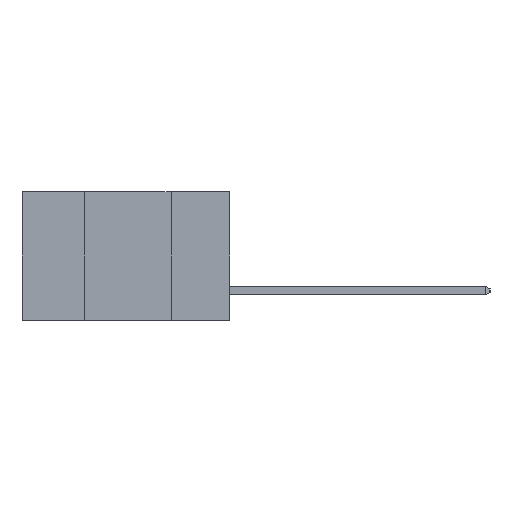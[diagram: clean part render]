
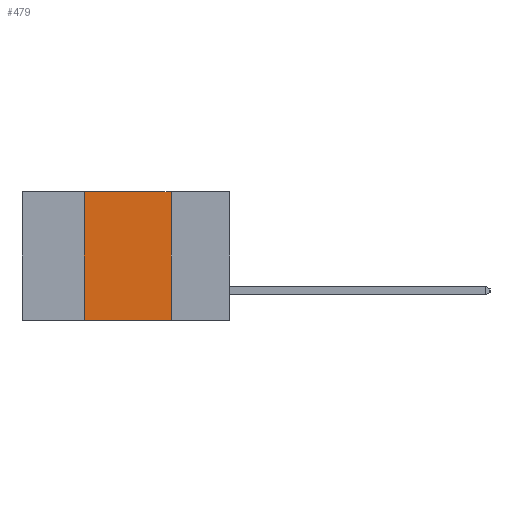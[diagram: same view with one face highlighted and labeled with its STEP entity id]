
A CAD part, left-side view. The second image highlights one B-rep face of the part: STEP entity #479.
In plain terms, the highlighted planar face has unit normal (-1, 0, 0).
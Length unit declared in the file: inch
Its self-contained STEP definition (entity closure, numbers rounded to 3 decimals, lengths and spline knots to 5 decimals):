
#479 = ADVANCED_FACE ( 'NONE', ( #17586 ), #18169, .F. ) ;
#842 = EDGE_CURVE ( 'NONE', #10505, #13944, #15516, .T. ) ;
#1056 = VECTOR ( 'NONE', #19393, 39.37008 ) ;
#1677 = VECTOR ( 'NONE', #4653, 39.37008 ) ;
#1993 = EDGE_CURVE ( 'NONE', #11078, #4246, #17641, .T. ) ;
#2008 = CARTESIAN_POINT ( 'NONE',  ( 0., 0.6, -0.37 ) ) ;
#3321 = EDGE_CURVE ( 'NONE', #10505, #11078, #14449, .T. ) ;
#3388 = ORIENTED_EDGE ( 'NONE', *, *, #8134, .F. ) ;
#4246 = VERTEX_POINT ( 'NONE', #14077 ) ;
#4653 = DIRECTION ( 'NONE',  ( 0., -1., 0. ) ) ;
#4935 = VECTOR ( 'NONE', #5342, 39.37008 ) ;
#5342 = DIRECTION ( 'NONE',  ( 0., 0., -1. ) ) ;
#5349 = CARTESIAN_POINT ( 'NONE',  ( 0., 0.17, 0. ) ) ;
#5687 = CARTESIAN_POINT ( 'NONE',  ( 0., 0.42, -0.37 ) ) ;
#6040 = CARTESIAN_POINT ( 'NONE',  ( 0., 0.6, 0. ) ) ;
#6084 = DIRECTION ( 'NONE',  ( 0., -1., 0. ) ) ;
#7272 = AXIS2_PLACEMENT_3D ( 'NONE', #14022, #17608, #15861 ) ;
#8134 = EDGE_CURVE ( 'NONE', #4246, #13944, #13514, .T. ) ;
#8153 = ORIENTED_EDGE ( 'NONE', *, *, #1993, .F. ) ;
#9238 = ORIENTED_EDGE ( 'NONE', *, *, #842, .T. ) ;
#10505 = VERTEX_POINT ( 'NONE', #5687 ) ;
#11043 = CARTESIAN_POINT ( 'NONE',  ( 0., 0.42, 0. ) ) ;
#11078 = VERTEX_POINT ( 'NONE', #15844 ) ;
#13514 = LINE ( 'NONE', #5349, #4935 ) ;
#13944 = VERTEX_POINT ( 'NONE', #20496 ) ;
#14022 = CARTESIAN_POINT ( 'NONE',  ( 0., 0.6, 0. ) ) ;
#14077 = CARTESIAN_POINT ( 'NONE',  ( 0., 0.17, 0. ) ) ;
#14449 = LINE ( 'NONE', #11043, #1056 ) ;
#15516 = LINE ( 'NONE', #2008, #1677 ) ;
#15844 = CARTESIAN_POINT ( 'NONE',  ( 0., 0.42, 0. ) ) ;
#15861 = DIRECTION ( 'NONE',  ( 0., 0., -1. ) ) ;
#16584 = VECTOR ( 'NONE', #6084, 39.37008 ) ;
#17586 = FACE_OUTER_BOUND ( 'NONE', #18292, .T. ) ;
#17608 = DIRECTION ( 'NONE',  ( 1., 0., 0. ) ) ;
#17641 = LINE ( 'NONE', #6040, #16584 ) ;
#18169 = PLANE ( 'NONE',  #7272 ) ;
#18292 = EDGE_LOOP ( 'NONE', ( #3388, #8153, #21375, #9238 ) ) ;
#19393 = DIRECTION ( 'NONE',  ( 0., 0., 1. ) ) ;
#20496 = CARTESIAN_POINT ( 'NONE',  ( 0., 0.17, -0.37 ) ) ;
#21375 = ORIENTED_EDGE ( 'NONE', *, *, #3321, .F. ) ;
